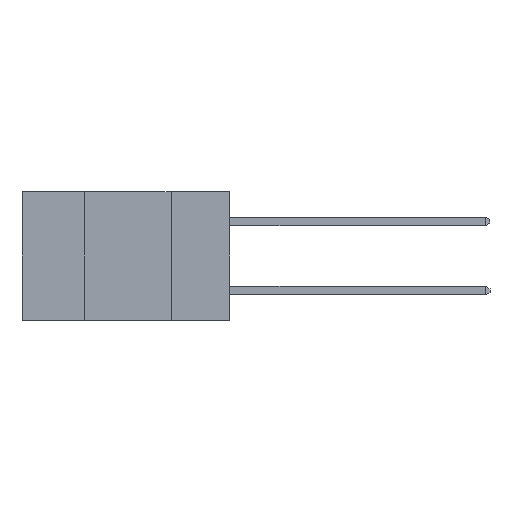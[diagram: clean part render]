
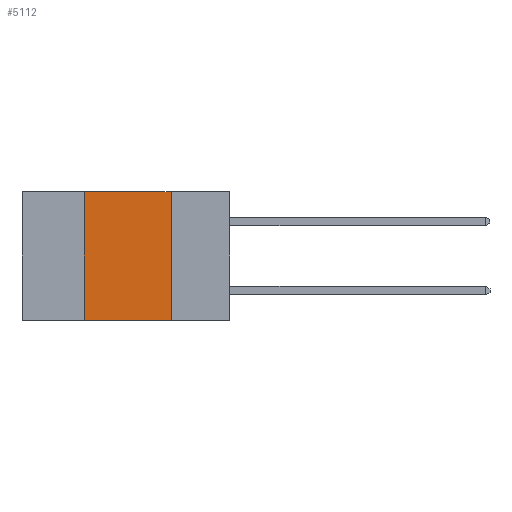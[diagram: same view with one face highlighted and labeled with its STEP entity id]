
A CAD part, left-side view. The second image highlights one B-rep face of the part: STEP entity #5112.
In plain terms, the highlighted planar face has unit normal (-1, 0, 0).
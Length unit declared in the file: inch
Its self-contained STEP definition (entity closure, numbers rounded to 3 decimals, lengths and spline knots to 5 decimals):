
#99 = VECTOR ( 'NONE', #4733, 39.37008 ) ;
#294 = PLANE ( 'NONE',  #1326 ) ;
#626 = CARTESIAN_POINT ( 'NONE',  ( 0., 0.6, 0. ) ) ;
#1326 = AXIS2_PLACEMENT_3D ( 'NONE', #10055, #7833, #2835 ) ;
#1487 = EDGE_LOOP ( 'NONE', ( #1517, #8637, #3598, #5165 ) ) ;
#1517 = ORIENTED_EDGE ( 'NONE', *, *, #3039, .F. ) ;
#1664 = EDGE_CURVE ( 'NONE', #9709, #4048, #8098, .T. ) ;
#1686 = VERTEX_POINT ( 'NONE', #8694 ) ;
#1922 = VERTEX_POINT ( 'NONE', #3366 ) ;
#2052 = LINE ( 'NONE', #5550, #10399 ) ;
#2130 = DIRECTION ( 'NONE',  ( 0., 0., -1. ) ) ;
#2389 = CARTESIAN_POINT ( 'NONE',  ( 0., 0.6, -0.37 ) ) ;
#2615 = LINE ( 'NONE', #626, #99 ) ;
#2835 = DIRECTION ( 'NONE',  ( 0., 0., -1. ) ) ;
#3039 = EDGE_CURVE ( 'NONE', #1922, #1686, #2052, .T. ) ;
#3366 = CARTESIAN_POINT ( 'NONE',  ( 0., 0.17, 0. ) ) ;
#3462 = FACE_OUTER_BOUND ( 'NONE', #1487, .T. ) ;
#3490 = EDGE_CURVE ( 'NONE', #9709, #1686, #7491, .T. ) ;
#3598 = ORIENTED_EDGE ( 'NONE', *, *, #1664, .F. ) ;
#4048 = VERTEX_POINT ( 'NONE', #7624 ) ;
#4733 = DIRECTION ( 'NONE',  ( 0., -1., 0. ) ) ;
#5112 = ADVANCED_FACE ( 'NONE', ( #3462 ), #294, .F. ) ;
#5165 = ORIENTED_EDGE ( 'NONE', *, *, #3490, .T. ) ;
#5550 = CARTESIAN_POINT ( 'NONE',  ( 0., 0.17, -0.37 ) ) ;
#5937 = VECTOR ( 'NONE', #7670, 39.37008 ) ;
#6501 = EDGE_CURVE ( 'NONE', #4048, #1922, #2615, .T. ) ;
#7254 = VECTOR ( 'NONE', #7715, 39.37008 ) ;
#7447 = CARTESIAN_POINT ( 'NONE',  ( 0., 0.42, -0.37 ) ) ;
#7491 = LINE ( 'NONE', #2389, #7254 ) ;
#7624 = CARTESIAN_POINT ( 'NONE',  ( 0., 0.42, 0. ) ) ;
#7670 = DIRECTION ( 'NONE',  ( 0., 0., 1. ) ) ;
#7715 = DIRECTION ( 'NONE',  ( 0., -1., 0. ) ) ;
#7833 = DIRECTION ( 'NONE',  ( 1., 0., 0. ) ) ;
#8098 = LINE ( 'NONE', #9434, #5937 ) ;
#8637 = ORIENTED_EDGE ( 'NONE', *, *, #6501, .F. ) ;
#8694 = CARTESIAN_POINT ( 'NONE',  ( 0., 0.17, -0.37 ) ) ;
#9434 = CARTESIAN_POINT ( 'NONE',  ( 0., 0.42, -0.37 ) ) ;
#9709 = VERTEX_POINT ( 'NONE', #7447 ) ;
#10055 = CARTESIAN_POINT ( 'NONE',  ( 0., 0.6, 0. ) ) ;
#10399 = VECTOR ( 'NONE', #2130, 39.37008 ) ;
